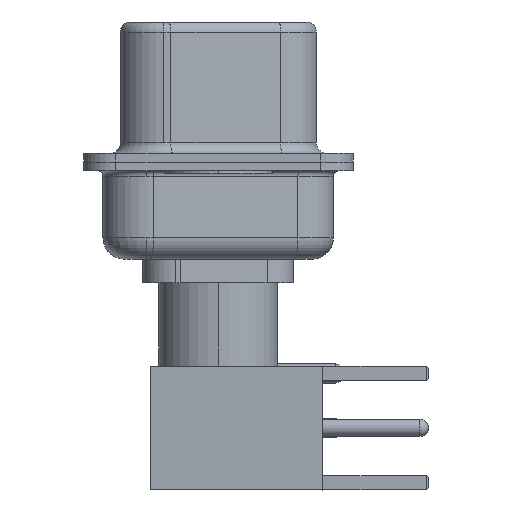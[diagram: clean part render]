
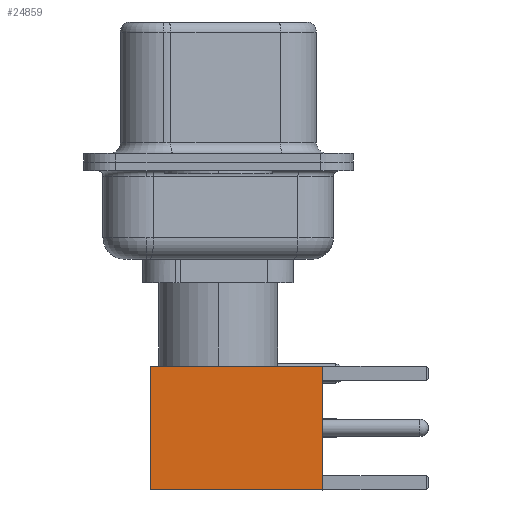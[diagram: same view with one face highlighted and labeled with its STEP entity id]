
A CAD part, left-side view. The second image highlights one B-rep face of the part: STEP entity #24859.
In plain terms, the highlighted face is planar.
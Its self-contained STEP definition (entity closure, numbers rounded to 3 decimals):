
#684 = VECTOR ( 'NONE', #3398, 1000. ) ;
#1851 = CARTESIAN_POINT ( 'NONE',  ( 2.875, 2.875, 0. ) ) ;
#2588 = CARTESIAN_POINT ( 'NONE',  ( 2.875, 2.875, 0. ) ) ;
#2911 = CARTESIAN_POINT ( 'NONE',  ( 0., 2.875, 0. ) ) ;
#3249 = CARTESIAN_POINT ( 'NONE',  ( 0., 2.875, 8. ) ) ;
#3293 = EDGE_CURVE ( 'NONE', #28681, #19441, #16705, .T. ) ;
#3398 = DIRECTION ( 'NONE',  ( -1., 0., 0. ) ) ;
#4585 = DIRECTION ( 'NONE',  ( 0., 0., -1. ) ) ;
#4700 = DIRECTION ( 'NONE',  ( 0., 1., 0. ) ) ;
#4868 = LINE ( 'NONE', #2588, #8746 ) ;
#4890 = VERTEX_POINT ( 'NONE', #17357 ) ;
#5604 = CARTESIAN_POINT ( 'NONE',  ( -2.875, 2.875, 8. ) ) ;
#7231 = FACE_OUTER_BOUND ( 'NONE', #25600, .T. ) ;
#8541 = LINE ( 'NONE', #3249, #684 ) ;
#8746 = VECTOR ( 'NONE', #4585, 1000. ) ;
#9057 = CARTESIAN_POINT ( 'NONE',  ( -2.875, 2.875, 0. ) ) ;
#9384 = PLANE ( 'NONE',  #24819 ) ;
#10753 = ORIENTED_EDGE ( 'NONE', *, *, #19114, .F. ) ;
#12005 = EDGE_CURVE ( 'NONE', #4890, #28681, #4868, .T. ) ;
#16258 = VECTOR ( 'NONE', #18308, 1000. ) ;
#16705 = LINE ( 'NONE', #2911, #21402 ) ;
#17357 = CARTESIAN_POINT ( 'NONE',  ( 2.875, 2.875, 8. ) ) ;
#18308 = DIRECTION ( 'NONE',  ( 0., 0., -1. ) ) ;
#19114 = EDGE_CURVE ( 'NONE', #28942, #19441, #29781, .T. ) ;
#19441 = VERTEX_POINT ( 'NONE', #24365 ) ;
#20907 = DIRECTION ( 'NONE',  ( 0., 0., 1. ) ) ;
#21058 = ORIENTED_EDGE ( 'NONE', *, *, #12005, .T. ) ;
#21084 = ORIENTED_EDGE ( 'NONE', *, *, #27981, .F. ) ;
#21402 = VECTOR ( 'NONE', #23676, 1000. ) ;
#23191 = ORIENTED_EDGE ( 'NONE', *, *, #3293, .T. ) ;
#23676 = DIRECTION ( 'NONE',  ( -1., 0., 0. ) ) ;
#24365 = CARTESIAN_POINT ( 'NONE',  ( -2.875, 2.875, 0. ) ) ;
#24819 = AXIS2_PLACEMENT_3D ( 'NONE', #25445, #4700, #20907 ) ;
#24859 = ADVANCED_FACE ( 'NONE', ( #7231 ), #9384, .T. ) ;
#25445 = CARTESIAN_POINT ( 'NONE',  ( 2.875, 2.875, 0. ) ) ;
#25600 = EDGE_LOOP ( 'NONE', ( #21058, #23191, #10753, #21084 ) ) ;
#27981 = EDGE_CURVE ( 'NONE', #4890, #28942, #8541, .T. ) ;
#28681 = VERTEX_POINT ( 'NONE', #1851 ) ;
#28942 = VERTEX_POINT ( 'NONE', #5604 ) ;
#29781 = LINE ( 'NONE', #9057, #16258 ) ;
